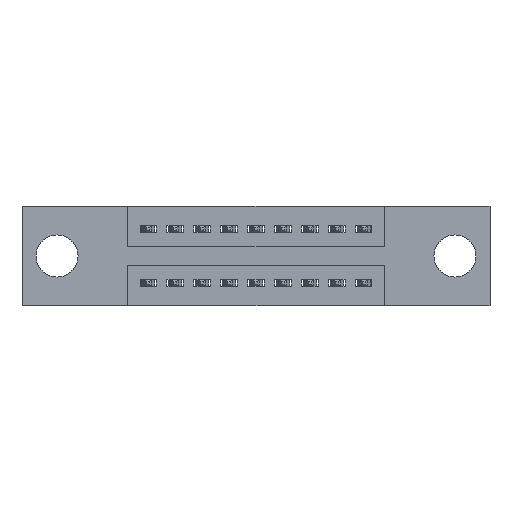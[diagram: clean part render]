
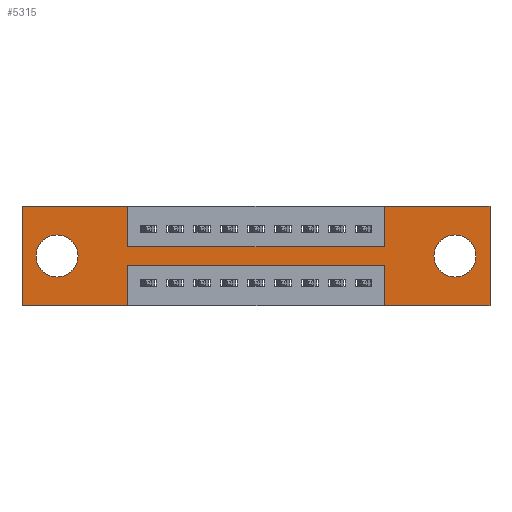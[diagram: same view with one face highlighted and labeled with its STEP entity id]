
A CAD part, front view. The second image highlights one B-rep face of the part: STEP entity #5315.
In plain terms, the highlighted planar face has unit normal (0, -1, 0).
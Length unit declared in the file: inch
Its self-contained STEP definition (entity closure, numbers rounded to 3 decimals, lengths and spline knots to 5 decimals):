
#20 = VERTEX_POINT ( 'NONE', #9077 ) ;
#32 = CARTESIAN_POINT ( 'NONE',  ( 0.3925, 0., -0.37 ) ) ;
#144 = ORIENTED_EDGE ( 'NONE', *, *, #6321, .F. ) ;
#299 = ORIENTED_EDGE ( 'NONE', *, *, #6871, .T. ) ;
#325 = VERTEX_POINT ( 'NONE', #7706 ) ;
#335 = DIRECTION ( 'NONE',  ( 1., 0., 0. ) ) ;
#392 = CARTESIAN_POINT ( 'NONE',  ( 0., 0., 0. ) ) ;
#456 = DIRECTION ( 'NONE',  ( 0., 0., -1. ) ) ;
#604 = ORIENTED_EDGE ( 'NONE', *, *, #11018, .T. ) ;
#634 = EDGE_CURVE ( 'NONE', #1644, #5132, #1769, .T. ) ;
#681 = CARTESIAN_POINT ( 'NONE',  ( 0., 0., -0.37 ) ) ;
#684 = VERTEX_POINT ( 'NONE', #11270 ) ;
#686 = LINE ( 'NONE', #2458, #3158 ) ;
#722 = VERTEX_POINT ( 'NONE', #10688 ) ;
#872 = CARTESIAN_POINT ( 'NONE',  ( 0.13, 0., -0.185 ) ) ;
#958 = CARTESIAN_POINT ( 'NONE',  ( 1.3425, 0., 0. ) ) ;
#965 = VERTEX_POINT ( 'NONE', #4773 ) ;
#1213 = EDGE_LOOP ( 'NONE', ( #10008, #8053, #6490, #9970, #144, #7772, #7080, #10972, #11175, #6104, #4260, #3479 ) ) ;
#1268 = CARTESIAN_POINT ( 'NONE',  ( 1.3425, 0., -0.37 ) ) ;
#1568 = VECTOR ( 'NONE', #456, 39.37008 ) ;
#1644 = VERTEX_POINT ( 'NONE', #8420 ) ;
#1657 = DIRECTION ( 'NONE',  ( 0., 0., 1. ) ) ;
#1716 = AXIS2_PLACEMENT_3D ( 'NONE', #9688, #10698, #1657 ) ;
#1724 = CARTESIAN_POINT ( 'NONE',  ( 1.735, 0., 0. ) ) ;
#1769 = CIRCLE ( 'NONE', #1716, 0.078 ) ;
#1810 = DIRECTION ( 'NONE',  ( 0., 0., 1. ) ) ;
#2101 = DIRECTION ( 'NONE',  ( 0., 0., 1. ) ) ;
#2178 = DIRECTION ( 'NONE',  ( 0., 0., 1. ) ) ;
#2458 = CARTESIAN_POINT ( 'NONE',  ( 0., 0., -0.37 ) ) ;
#2492 = DIRECTION ( 'NONE',  ( 0., 1., 0. ) ) ;
#2550 = CARTESIAN_POINT ( 'NONE',  ( 1.605, 0., -0.107 ) ) ;
#2577 = VECTOR ( 'NONE', #9759, 39.37008 ) ;
#2605 = VERTEX_POINT ( 'NONE', #958 ) ;
#2643 = DIRECTION ( 'NONE',  ( 1., 0., 0. ) ) ;
#2691 = DIRECTION ( 'NONE',  ( 1., 0., 0. ) ) ;
#2758 = FACE_BOUND ( 'NONE', #9125, .T. ) ;
#2815 = AXIS2_PLACEMENT_3D ( 'NONE', #8997, #3523, #9806 ) ;
#2848 = LINE ( 'NONE', #3050, #7554 ) ;
#3050 = CARTESIAN_POINT ( 'NONE',  ( 1.3425, 0., 0. ) ) ;
#3105 = EDGE_LOOP ( 'NONE', ( #6271, #8566 ) ) ;
#3158 = VECTOR ( 'NONE', #8074, 39.37008 ) ;
#3165 = CARTESIAN_POINT ( 'NONE',  ( 0., 0., 0. ) ) ;
#3479 = ORIENTED_EDGE ( 'NONE', *, *, #6429, .F. ) ;
#3523 = DIRECTION ( 'NONE',  ( 0., 1., 0. ) ) ;
#3735 = CARTESIAN_POINT ( 'NONE',  ( 0., 0., -0.37 ) ) ;
#4004 = LINE ( 'NONE', #7301, #8597 ) ;
#4260 = ORIENTED_EDGE ( 'NONE', *, *, #6252, .F. ) ;
#4454 = VECTOR ( 'NONE', #2178, 39.37008 ) ;
#4484 = CARTESIAN_POINT ( 'NONE',  ( 0.3925, 0., -0.15 ) ) ;
#4609 = CIRCLE ( 'NONE', #2815, 0.078 ) ;
#4640 = EDGE_CURVE ( 'NONE', #9705, #6463, #9347, .T. ) ;
#4773 = CARTESIAN_POINT ( 'NONE',  ( 0.3925, 0., -0.22 ) ) ;
#4775 = LINE ( 'NONE', #681, #2577 ) ;
#4799 = VERTEX_POINT ( 'NONE', #1724 ) ;
#4879 = CARTESIAN_POINT ( 'NONE',  ( 0., 0., 0. ) ) ;
#4918 = LINE ( 'NONE', #3165, #9668 ) ;
#5132 = VERTEX_POINT ( 'NONE', #8780 ) ;
#5315 = ADVANCED_FACE ( 'NONE', ( #2758, #9204, #11036 ), #11265, .T. ) ;
#5319 = VERTEX_POINT ( 'NONE', #11417 ) ;
#5463 = AXIS2_PLACEMENT_3D ( 'NONE', #8099, #2492, #8933 ) ;
#5671 = CARTESIAN_POINT ( 'NONE',  ( 0., 0., -0.37 ) ) ;
#5771 = DIRECTION ( 'NONE',  ( 0., 0., -1. ) ) ;
#5876 = EDGE_CURVE ( 'NONE', #2605, #4799, #7317, .T. ) ;
#5928 = VECTOR ( 'NONE', #5771, 39.37008 ) ;
#6104 = ORIENTED_EDGE ( 'NONE', *, *, #4640, .F. ) ;
#6223 = LINE ( 'NONE', #4484, #10258 ) ;
#6252 = EDGE_CURVE ( 'NONE', #7093, #9705, #4918, .T. ) ;
#6271 = ORIENTED_EDGE ( 'NONE', *, *, #7056, .T. ) ;
#6321 = EDGE_CURVE ( 'NONE', #4799, #5319, #11250, .T. ) ;
#6390 = EDGE_CURVE ( 'NONE', #5319, #8146, #686, .T. ) ;
#6407 = CARTESIAN_POINT ( 'NONE',  ( 0.3925, 0., 0. ) ) ;
#6429 = EDGE_CURVE ( 'NONE', #9753, #7093, #4775, .T. ) ;
#6442 = VERTEX_POINT ( 'NONE', #2550 ) ;
#6463 = VERTEX_POINT ( 'NONE', #6407 ) ;
#6490 = ORIENTED_EDGE ( 'NONE', *, *, #7891, .F. ) ;
#6663 = AXIS2_PLACEMENT_3D ( 'NONE', #5671, #11296, #11366 ) ;
#6772 = CARTESIAN_POINT ( 'NONE',  ( 0.3925, 0., -0.22 ) ) ;
#6871 = EDGE_CURVE ( 'NONE', #6442, #722, #10286, .T. ) ;
#7056 = EDGE_CURVE ( 'NONE', #5132, #1644, #10891, .T. ) ;
#7060 = CARTESIAN_POINT ( 'NONE',  ( 1.735, 0., 0. ) ) ;
#7080 = ORIENTED_EDGE ( 'NONE', *, *, #7843, .F. ) ;
#7093 = VERTEX_POINT ( 'NONE', #3735 ) ;
#7233 = EDGE_CURVE ( 'NONE', #325, #965, #7707, .T. ) ;
#7301 = CARTESIAN_POINT ( 'NONE',  ( 0.3925, 0., 0. ) ) ;
#7317 = LINE ( 'NONE', #392, #9552 ) ;
#7451 = DIRECTION ( 'NONE',  ( 0., 1., 0. ) ) ;
#7554 = VECTOR ( 'NONE', #2101, 39.37008 ) ;
#7706 = CARTESIAN_POINT ( 'NONE',  ( 1.3425, 0., -0.22 ) ) ;
#7707 = LINE ( 'NONE', #6772, #11467 ) ;
#7772 = ORIENTED_EDGE ( 'NONE', *, *, #5876, .F. ) ;
#7788 = EDGE_CURVE ( 'NONE', #965, #9753, #8371, .T. ) ;
#7843 = EDGE_CURVE ( 'NONE', #684, #2605, #2848, .T. ) ;
#7891 = EDGE_CURVE ( 'NONE', #8146, #325, #9514, .T. ) ;
#8053 = ORIENTED_EDGE ( 'NONE', *, *, #7233, .F. ) ;
#8074 = DIRECTION ( 'NONE',  ( -1., 0., 0. ) ) ;
#8099 = CARTESIAN_POINT ( 'NONE',  ( 1.605, 0., -0.185 ) ) ;
#8146 = VERTEX_POINT ( 'NONE', #9723 ) ;
#8176 = DIRECTION ( 'NONE',  ( 0., 0., -1. ) ) ;
#8245 = EDGE_CURVE ( 'NONE', #6463, #20, #4004, .T. ) ;
#8261 = EDGE_CURVE ( 'NONE', #20, #684, #6223, .T. ) ;
#8371 = LINE ( 'NONE', #10110, #5928 ) ;
#8420 = CARTESIAN_POINT ( 'NONE',  ( 0.13, 0., -0.263 ) ) ;
#8524 = DIRECTION ( 'NONE',  ( -1., 0., 0. ) ) ;
#8566 = ORIENTED_EDGE ( 'NONE', *, *, #634, .T. ) ;
#8597 = VECTOR ( 'NONE', #8176, 39.37008 ) ;
#8780 = CARTESIAN_POINT ( 'NONE',  ( 0.13, 0., -0.107 ) ) ;
#8933 = DIRECTION ( 'NONE',  ( 0., 0., -1. ) ) ;
#8997 = CARTESIAN_POINT ( 'NONE',  ( 1.605, 0., -0.185 ) ) ;
#9077 = CARTESIAN_POINT ( 'NONE',  ( 0.3925, 0., -0.15 ) ) ;
#9125 = EDGE_LOOP ( 'NONE', ( #299, #604 ) ) ;
#9204 = FACE_BOUND ( 'NONE', #3105, .T. ) ;
#9347 = LINE ( 'NONE', #4879, #11162 ) ;
#9514 = LINE ( 'NONE', #1268, #4454 ) ;
#9552 = VECTOR ( 'NONE', #335, 39.37008 ) ;
#9668 = VECTOR ( 'NONE', #11088, 39.37008 ) ;
#9688 = CARTESIAN_POINT ( 'NONE',  ( 0.13, 0., -0.185 ) ) ;
#9705 = VERTEX_POINT ( 'NONE', #10003 ) ;
#9723 = CARTESIAN_POINT ( 'NONE',  ( 1.3425, 0., -0.37 ) ) ;
#9753 = VERTEX_POINT ( 'NONE', #32 ) ;
#9759 = DIRECTION ( 'NONE',  ( -1., 0., 0. ) ) ;
#9806 = DIRECTION ( 'NONE',  ( 0., 0., -1. ) ) ;
#9970 = ORIENTED_EDGE ( 'NONE', *, *, #6390, .F. ) ;
#10003 = CARTESIAN_POINT ( 'NONE',  ( 0., 0., 0. ) ) ;
#10008 = ORIENTED_EDGE ( 'NONE', *, *, #7788, .F. ) ;
#10110 = CARTESIAN_POINT ( 'NONE',  ( 0.3925, 0., -0.37 ) ) ;
#10258 = VECTOR ( 'NONE', #2643, 39.37008 ) ;
#10286 = CIRCLE ( 'NONE', #5463, 0.078 ) ;
#10688 = CARTESIAN_POINT ( 'NONE',  ( 1.605, 0., -0.263 ) ) ;
#10698 = DIRECTION ( 'NONE',  ( 0., 1., 0. ) ) ;
#10891 = CIRCLE ( 'NONE', #11171, 0.078 ) ;
#10972 = ORIENTED_EDGE ( 'NONE', *, *, #8261, .F. ) ;
#11018 = EDGE_CURVE ( 'NONE', #722, #6442, #4609, .T. ) ;
#11036 = FACE_OUTER_BOUND ( 'NONE', #1213, .T. ) ;
#11088 = DIRECTION ( 'NONE',  ( 0., 0., 1. ) ) ;
#11162 = VECTOR ( 'NONE', #2691, 39.37008 ) ;
#11171 = AXIS2_PLACEMENT_3D ( 'NONE', #872, #7451, #1810 ) ;
#11175 = ORIENTED_EDGE ( 'NONE', *, *, #8245, .F. ) ;
#11250 = LINE ( 'NONE', #7060, #1568 ) ;
#11265 = PLANE ( 'NONE',  #6663 ) ;
#11270 = CARTESIAN_POINT ( 'NONE',  ( 1.3425, 0., -0.15 ) ) ;
#11296 = DIRECTION ( 'NONE',  ( 0., -1., 0. ) ) ;
#11366 = DIRECTION ( 'NONE',  ( 0., 0., -1. ) ) ;
#11417 = CARTESIAN_POINT ( 'NONE',  ( 1.735, 0., -0.37 ) ) ;
#11467 = VECTOR ( 'NONE', #8524, 39.37008 ) ;
